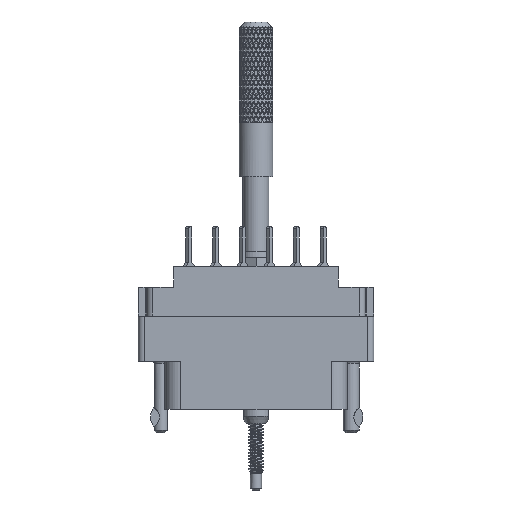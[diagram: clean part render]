
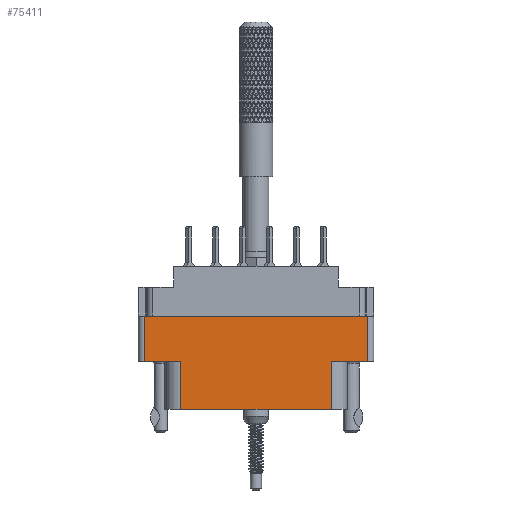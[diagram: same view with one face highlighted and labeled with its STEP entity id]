
A CAD part, front view. The second image highlights one B-rep face of the part: STEP entity #75411.
In plain terms, the highlighted planar face has unit normal (0, -1, 0).
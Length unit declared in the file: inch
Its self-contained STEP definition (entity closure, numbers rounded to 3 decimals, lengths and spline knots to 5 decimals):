
#1360 = EDGE_CURVE ( 'NONE', #110372, #37374, #74816, .T. ) ;
#1774 = VERTEX_POINT ( 'NONE', #97898 ) ;
#15524 = EDGE_CURVE ( 'NONE', #126628, #177259, #107906, .T. ) ;
#17460 = LINE ( 'NONE', #29560, #73222 ) ;
#21236 = CARTESIAN_POINT ( 'NONE',  ( -0.42, -0.343, -0.798 ) ) ;
#23703 = ORIENTED_EDGE ( 'NONE', *, *, #42040, .T. ) ;
#26120 = DIRECTION ( 'NONE',  ( -1., 0., 0. ) ) ;
#26867 = VECTOR ( 'NONE', #136985, 39.37008 ) ;
#29560 = CARTESIAN_POINT ( 'NONE',  ( 0.624, -0.343, -0.798 ) ) ;
#29825 = DIRECTION ( 'NONE',  ( 1., 0., 0. ) ) ;
#32149 = DIRECTION ( 'NONE',  ( 0., -1., 0. ) ) ;
#32499 = ORIENTED_EDGE ( 'NONE', *, *, #188428, .F. ) ;
#33578 = DIRECTION ( 'NONE',  ( 1., 0., 0. ) ) ;
#34571 = CARTESIAN_POINT ( 'NONE',  ( 0.624, -0.343, -0.529 ) ) ;
#35226 = VECTOR ( 'NONE', #72611, 39.37008 ) ;
#37374 = VERTEX_POINT ( 'NONE', #21236 ) ;
#42040 = EDGE_CURVE ( 'NONE', #151931, #110372, #116412, .T. ) ;
#46406 = PLANE ( 'NONE',  #124600 ) ;
#51438 = EDGE_CURVE ( 'NONE', #191601, #126628, #154691, .T. ) ;
#55675 = EDGE_CURVE ( 'NONE', #1774, #140667, #147024, .T. ) ;
#70617 = VECTOR ( 'NONE', #182259, 39.37008 ) ;
#70674 = CARTESIAN_POINT ( 'NONE',  ( -0.42, -0.343, -0.529 ) ) ;
#72216 = CARTESIAN_POINT ( 'NONE',  ( 0., -0.343, -0.529 ) ) ;
#72611 = DIRECTION ( 'NONE',  ( 0., 0., -1. ) ) ;
#73222 = VECTOR ( 'NONE', #151251, 39.37008 ) ;
#74816 = LINE ( 'NONE', #70674, #35226 ) ;
#75411 = ADVANCED_FACE ( 'NONE', ( #139053 ), #46406, .T. ) ;
#76380 = CARTESIAN_POINT ( 'NONE',  ( -0.624, -0.343, -0.798 ) ) ;
#77244 = ORIENTED_EDGE ( 'NONE', *, *, #55675, .F. ) ;
#82693 = CARTESIAN_POINT ( 'NONE',  ( 0.42, -0.343, -0.798 ) ) ;
#84805 = VECTOR ( 'NONE', #26120, 39.37008 ) ;
#86236 = VECTOR ( 'NONE', #29825, 39.37008 ) ;
#87760 = CARTESIAN_POINT ( 'NONE',  ( 0., -0.343, -0.529 ) ) ;
#88949 = DIRECTION ( 'NONE',  ( 0., 0., 1. ) ) ;
#89479 = ORIENTED_EDGE ( 'NONE', *, *, #15524, .F. ) ;
#90132 = ORIENTED_EDGE ( 'NONE', *, *, #185044, .T. ) ;
#95607 = ORIENTED_EDGE ( 'NONE', *, *, #51438, .F. ) ;
#97141 = CARTESIAN_POINT ( 'NONE',  ( -0.42, -0.343, -0.529 ) ) ;
#97898 = CARTESIAN_POINT ( 'NONE',  ( -0.624, -0.343, -0.277 ) ) ;
#103283 = CARTESIAN_POINT ( 'NONE',  ( -0.624, -0.343, -0.798 ) ) ;
#107906 = LINE ( 'NONE', #133419, #70617 ) ;
#108455 = ORIENTED_EDGE ( 'NONE', *, *, #108826, .T. ) ;
#108826 = EDGE_CURVE ( 'NONE', #37374, #177259, #159641, .T. ) ;
#110372 = VERTEX_POINT ( 'NONE', #97141 ) ;
#116412 = LINE ( 'NONE', #87760, #86236 ) ;
#121967 = CARTESIAN_POINT ( 'NONE',  ( -0.624, -0.343, -0.798 ) ) ;
#123861 = VECTOR ( 'NONE', #88949, 39.37008 ) ;
#124600 = AXIS2_PLACEMENT_3D ( 'NONE', #76380, #32149, #152579 ) ;
#126628 = VERTEX_POINT ( 'NONE', #170185 ) ;
#133254 = LINE ( 'NONE', #103283, #123861 ) ;
#133419 = CARTESIAN_POINT ( 'NONE',  ( 0.42, -0.343, -0.529 ) ) ;
#136773 = CARTESIAN_POINT ( 'NONE',  ( 0.624, -0.343, -0.277 ) ) ;
#136985 = DIRECTION ( 'NONE',  ( 1., 0., 0. ) ) ;
#139053 = FACE_OUTER_BOUND ( 'NONE', #151043, .T. ) ;
#140667 = VERTEX_POINT ( 'NONE', #136773 ) ;
#147024 = LINE ( 'NONE', #182618, #174839 ) ;
#150646 = CARTESIAN_POINT ( 'NONE',  ( -0.624, -0.343, -0.529 ) ) ;
#151043 = EDGE_LOOP ( 'NONE', ( #192138, #108455, #89479, #95607, #90132, #77244, #32499, #23703 ) ) ;
#151251 = DIRECTION ( 'NONE',  ( 0., 0., 1. ) ) ;
#151931 = VERTEX_POINT ( 'NONE', #150646 ) ;
#152579 = DIRECTION ( 'NONE',  ( 0., 0., -1. ) ) ;
#154691 = LINE ( 'NONE', #72216, #84805 ) ;
#159641 = LINE ( 'NONE', #121967, #26867 ) ;
#170185 = CARTESIAN_POINT ( 'NONE',  ( 0.42, -0.343, -0.529 ) ) ;
#174839 = VECTOR ( 'NONE', #33578, 39.37008 ) ;
#177259 = VERTEX_POINT ( 'NONE', #82693 ) ;
#182259 = DIRECTION ( 'NONE',  ( 0., 0., -1. ) ) ;
#182618 = CARTESIAN_POINT ( 'NONE',  ( -0.656, -0.343, -0.277 ) ) ;
#185044 = EDGE_CURVE ( 'NONE', #191601, #140667, #17460, .T. ) ;
#188428 = EDGE_CURVE ( 'NONE', #151931, #1774, #133254, .T. ) ;
#191601 = VERTEX_POINT ( 'NONE', #34571 ) ;
#192138 = ORIENTED_EDGE ( 'NONE', *, *, #1360, .T. ) ;
